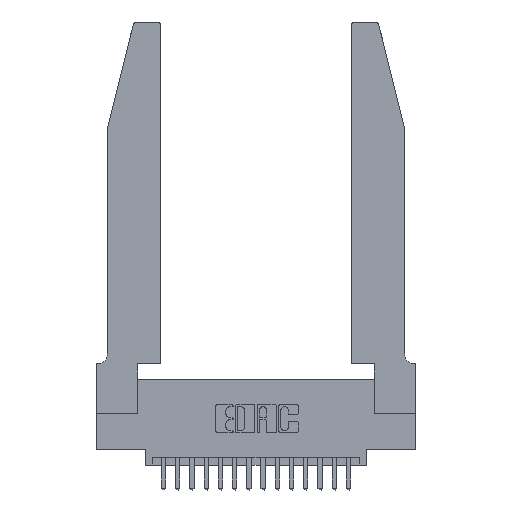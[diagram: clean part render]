
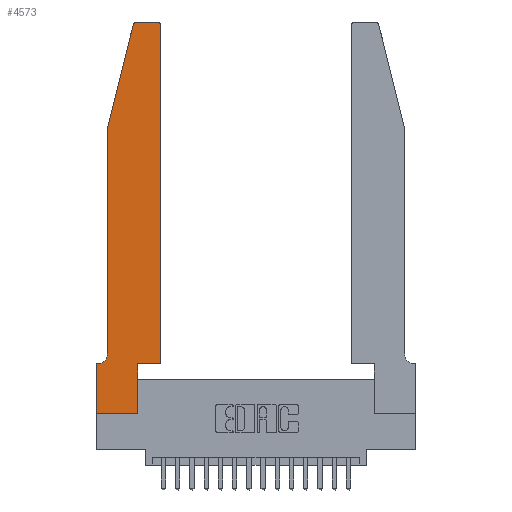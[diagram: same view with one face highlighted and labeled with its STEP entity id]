
A CAD part, top view. The second image highlights one B-rep face of the part: STEP entity #4573.
In plain terms, the highlighted planar face has unit normal (0, 0, 1).
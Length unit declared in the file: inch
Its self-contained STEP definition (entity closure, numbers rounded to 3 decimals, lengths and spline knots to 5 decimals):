
#283 = ORIENTED_EDGE ( 'NONE', *, *, #5945, .T. ) ;
#426 = AXIS2_PLACEMENT_3D ( 'NONE', #4614, #15156, #6144 ) ;
#591 = VECTOR ( 'NONE', #5802, 39.37008 ) ;
#650 = CARTESIAN_POINT ( 'NONE',  ( 0., 0., 0.37 ) ) ;
#912 = DIRECTION ( 'NONE',  ( 1., 0., 0. ) ) ;
#1128 = VERTEX_POINT ( 'NONE', #14366 ) ;
#1166 = DIRECTION ( 'NONE',  ( 0., 1., 0. ) ) ;
#2213 = ORIENTED_EDGE ( 'NONE', *, *, #10010, .T. ) ;
#2331 = LINE ( 'NONE', #19360, #6461 ) ;
#2631 = CARTESIAN_POINT ( 'NONE',  ( 0.2865, 0.35, 0.37 ) ) ;
#2894 = DIRECTION ( 'NONE',  ( 1., 0., 0. ) ) ;
#3044 = CARTESIAN_POINT ( 'NONE',  ( 0.25487, 2.72718, 0.37 ) ) ;
#3300 = CARTESIAN_POINT ( 'NONE',  ( 0.2865, 0., 0.37 ) ) ;
#3302 = CARTESIAN_POINT ( 'NONE',  ( 0.0755, 2., 0.37 ) ) ;
#3409 = CIRCLE ( 'NONE', #5521, 0.03 ) ;
#3416 = CIRCLE ( 'NONE', #6312, 0.07 ) ;
#3430 = DIRECTION ( 'NONE',  ( -1., 0., 0. ) ) ;
#3438 = DIRECTION ( 'NONE',  ( -1., 0., 0. ) ) ;
#4429 = EDGE_CURVE ( 'NONE', #8313, #16960, #19503, .T. ) ;
#4473 = CARTESIAN_POINT ( 'NONE',  ( 0.4505, 0.35, 0.37 ) ) ;
#4573 = ADVANCED_FACE ( 'NONE', ( #16881 ), #11612, .T. ) ;
#4614 = CARTESIAN_POINT ( 'NONE',  ( 0.284, 2.72, 0.37 ) ) ;
#4815 = LINE ( 'NONE', #13292, #591 ) ;
#4933 = EDGE_CURVE ( 'NONE', #15774, #6946, #17803, .T. ) ;
#4946 = ORIENTED_EDGE ( 'NONE', *, *, #4429, .T. ) ;
#5095 = EDGE_CURVE ( 'NONE', #11098, #6278, #3416, .T. ) ;
#5170 = CARTESIAN_POINT ( 'NONE',  ( 0., 0., 0.37 ) ) ;
#5269 = CARTESIAN_POINT ( 'NONE',  ( 0.4505, 2.72, 0.37 ) ) ;
#5418 = VECTOR ( 'NONE', #17439, 39.37008 ) ;
#5438 = CARTESIAN_POINT ( 'NONE',  ( 0.0055, 0.42, 0.37 ) ) ;
#5521 = AXIS2_PLACEMENT_3D ( 'NONE', #7274, #17750, #8770 ) ;
#5802 = DIRECTION ( 'NONE',  ( 0., -1., 0. ) ) ;
#5880 = CARTESIAN_POINT ( 'NONE',  ( 0.0755, 0.42, 0.37 ) ) ;
#5945 = EDGE_CURVE ( 'NONE', #13906, #1128, #13326, .T. ) ;
#6144 = DIRECTION ( 'NONE',  ( 1., 0., 0. ) ) ;
#6278 = VERTEX_POINT ( 'NONE', #17356 ) ;
#6312 = AXIS2_PLACEMENT_3D ( 'NONE', #5438, #15959, #6971 ) ;
#6390 = EDGE_CURVE ( 'NONE', #16960, #11098, #4815, .T. ) ;
#6461 = VECTOR ( 'NONE', #1166, 39.37008 ) ;
#6797 = CARTESIAN_POINT ( 'NONE',  ( 0.0755, 2., 0.37 ) ) ;
#6946 = VERTEX_POINT ( 'NONE', #13143 ) ;
#6971 = DIRECTION ( 'NONE',  ( -1., 0., 0. ) ) ;
#7031 = EDGE_CURVE ( 'NONE', #1128, #17126, #2331, .T. ) ;
#7167 = VECTOR ( 'NONE', #3438, 39.37008 ) ;
#7274 = CARTESIAN_POINT ( 'NONE',  ( 0.4205, 2.72, 0.37 ) ) ;
#7455 = LINE ( 'NONE', #9897, #15449 ) ;
#7872 = VERTEX_POINT ( 'NONE', #3300 ) ;
#7949 = EDGE_CURVE ( 'NONE', #6278, #8637, #19130, .T. ) ;
#8030 = CARTESIAN_POINT ( 'NONE',  ( 0.2605, 2.75, 0.37 ) ) ;
#8042 = CARTESIAN_POINT ( 'NONE',  ( 0.0755, 0.35, 0.37 ) ) ;
#8313 = VERTEX_POINT ( 'NONE', #3044 ) ;
#8637 = VERTEX_POINT ( 'NONE', #11369 ) ;
#8770 = DIRECTION ( 'NONE',  ( 1., 0., 0. ) ) ;
#8853 = VECTOR ( 'NONE', #2894, 39.37008 ) ;
#9007 = ORIENTED_EDGE ( 'NONE', *, *, #5095, .T. ) ;
#9200 = CIRCLE ( 'NONE', #426, 0.03 ) ;
#9446 = LINE ( 'NONE', #650, #5418 ) ;
#9750 = LINE ( 'NONE', #2631, #14191 ) ;
#9897 = CARTESIAN_POINT ( 'NONE',  ( 0., 0., 0.37 ) ) ;
#10010 = EDGE_CURVE ( 'NONE', #6946, #8313, #9200, .T. ) ;
#10160 = DIRECTION ( 'NONE',  ( 0., 0., 1. ) ) ;
#11098 = VERTEX_POINT ( 'NONE', #5880 ) ;
#11369 = CARTESIAN_POINT ( 'NONE',  ( 0., 0.35, 0.37 ) ) ;
#11557 = VECTOR ( 'NONE', #15797, 39.37008 ) ;
#11612 = PLANE ( 'NONE',  #14106 ) ;
#12078 = VERTEX_POINT ( 'NONE', #5170 ) ;
#12286 = EDGE_CURVE ( 'NONE', #7872, #13906, #9750, .T. ) ;
#12363 = ORIENTED_EDGE ( 'NONE', *, *, #6390, .T. ) ;
#12815 = EDGE_LOOP ( 'NONE', ( #14123, #2213, #4946, #12363, #9007, #13233, #13562, #17761, #15199, #283, #13596, #13644 ) ) ;
#13143 = CARTESIAN_POINT ( 'NONE',  ( 0.284, 2.75, 0.37 ) ) ;
#13233 = ORIENTED_EDGE ( 'NONE', *, *, #7949, .T. ) ;
#13292 = CARTESIAN_POINT ( 'NONE',  ( 0.0755, 2., 0.37 ) ) ;
#13326 = LINE ( 'NONE', #4473, #8853 ) ;
#13359 = VECTOR ( 'NONE', #3430, 39.37008 ) ;
#13562 = ORIENTED_EDGE ( 'NONE', *, *, #13900, .T. ) ;
#13596 = ORIENTED_EDGE ( 'NONE', *, *, #7031, .T. ) ;
#13644 = ORIENTED_EDGE ( 'NONE', *, *, #16680, .T. ) ;
#13900 = EDGE_CURVE ( 'NONE', #8637, #12078, #9446, .T. ) ;
#13906 = VERTEX_POINT ( 'NONE', #15941 ) ;
#14106 = AXIS2_PLACEMENT_3D ( 'NONE', #19123, #10160, #912 ) ;
#14123 = ORIENTED_EDGE ( 'NONE', *, *, #4933, .T. ) ;
#14191 = VECTOR ( 'NONE', #17698, 39.37008 ) ;
#14366 = CARTESIAN_POINT ( 'NONE',  ( 0.4505, 0.35, 0.37 ) ) ;
#14758 = CARTESIAN_POINT ( 'NONE',  ( 0.4205, 2.75, 0.37 ) ) ;
#15156 = DIRECTION ( 'NONE',  ( 0., 0., 1. ) ) ;
#15199 = ORIENTED_EDGE ( 'NONE', *, *, #12286, .T. ) ;
#15449 = VECTOR ( 'NONE', #18859, 39.37008 ) ;
#15774 = VERTEX_POINT ( 'NONE', #14758 ) ;
#15797 = DIRECTION ( 'NONE',  ( -0.239, -0.971, 0. ) ) ;
#15941 = CARTESIAN_POINT ( 'NONE',  ( 0.2865, 0.35, 0.37 ) ) ;
#15959 = DIRECTION ( 'NONE',  ( 0., 0., -1. ) ) ;
#16680 = EDGE_CURVE ( 'NONE', #17126, #15774, #3409, .T. ) ;
#16881 = FACE_OUTER_BOUND ( 'NONE', #12815, .T. ) ;
#16960 = VERTEX_POINT ( 'NONE', #3302 ) ;
#17126 = VERTEX_POINT ( 'NONE', #5269 ) ;
#17165 = EDGE_CURVE ( 'NONE', #12078, #7872, #7455, .T. ) ;
#17356 = CARTESIAN_POINT ( 'NONE',  ( 0.0055, 0.35, 0.37 ) ) ;
#17439 = DIRECTION ( 'NONE',  ( 0., -1., 0. ) ) ;
#17698 = DIRECTION ( 'NONE',  ( 0., 1., 0. ) ) ;
#17750 = DIRECTION ( 'NONE',  ( 0., 0., 1. ) ) ;
#17761 = ORIENTED_EDGE ( 'NONE', *, *, #17165, .T. ) ;
#17803 = LINE ( 'NONE', #8030, #13359 ) ;
#18859 = DIRECTION ( 'NONE',  ( 1., 0., 0. ) ) ;
#19123 = CARTESIAN_POINT ( 'NONE',  ( 0., 0.35, 0.37 ) ) ;
#19130 = LINE ( 'NONE', #8042, #7167 ) ;
#19360 = CARTESIAN_POINT ( 'NONE',  ( 0.4505, 0.35, 0.37 ) ) ;
#19503 = LINE ( 'NONE', #6797, #11557 ) ;
